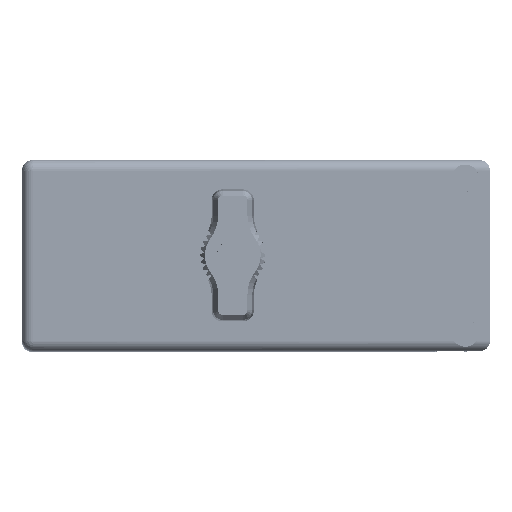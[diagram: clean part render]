
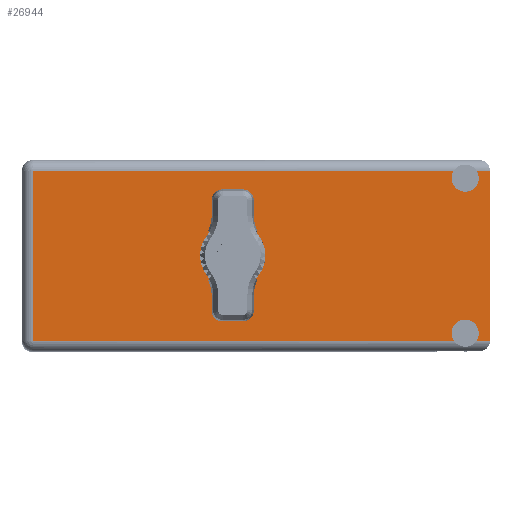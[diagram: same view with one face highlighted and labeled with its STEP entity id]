
A CAD part, top view. The second image highlights one B-rep face of the part: STEP entity #26944.
In plain terms, the highlighted face is planar.
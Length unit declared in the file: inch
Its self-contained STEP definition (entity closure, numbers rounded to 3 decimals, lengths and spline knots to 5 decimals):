
#240 = ORIENTED_EDGE ( 'NONE', *, *, #15233, .F. ) ;
#1198 = CARTESIAN_POINT ( 'NONE',  ( 1.42519, 1.675, -0.547 ) ) ;
#1617 = CARTESIAN_POINT ( 'NONE',  ( 1.499, 1.675, 0.5 ) ) ;
#3322 = CARTESIAN_POINT ( 'NONE',  ( 1.499, 1.675, -0.5 ) ) ;
#3439 = ORIENTED_EDGE ( 'NONE', *, *, #83139, .F. ) ;
#4769 = CARTESIAN_POINT ( 'NONE',  ( 1.659, 1.675, 0.617 ) ) ;
#5890 = LINE ( 'NONE', #4769, #50999 ) ;
#5901 = CARTESIAN_POINT ( 'NONE',  ( 1.42519, 1.675, 0.547 ) ) ;
#5935 = EDGE_CURVE ( 'NONE', #7246, #65026, #33820, .T. ) ;
#6050 = CARTESIAN_POINT ( 'NONE',  ( 0., 1.675, 0.125 ) ) ;
#7246 = VERTEX_POINT ( 'NONE', #82256 ) ;
#9807 = CARTESIAN_POINT ( 'NONE',  ( 1.499, 1.675, -0.4125 ) ) ;
#10256 = PLANE ( 'NONE',  #47088 ) ;
#10401 = DIRECTION ( 'NONE',  ( 0., 1., 0. ) ) ;
#10644 = VECTOR ( 'NONE', #65956, 39.37008 ) ;
#11143 = CARTESIAN_POINT ( 'NONE',  ( 1.659, 1.675, 0.547 ) ) ;
#11753 = DIRECTION ( 'NONE',  ( 0., 1., 0. ) ) ;
#13072 = CIRCLE ( 'NONE', #24403, 0.0875 ) ;
#14106 = DIRECTION ( 'NONE',  ( 0., 0., 1. ) ) ;
#14936 = CARTESIAN_POINT ( 'NONE',  ( -1.289, 1.675, -0.617 ) ) ;
#15233 = EDGE_CURVE ( 'NONE', #57375, #23642, #34557, .T. ) ;
#15489 = CARTESIAN_POINT ( 'NONE',  ( 1.659, 1.675, -0.547 ) ) ;
#16660 = DIRECTION ( 'NONE',  ( 1., 0., 0. ) ) ;
#16990 = CARTESIAN_POINT ( 'NONE',  ( -1.359, 1.675, -0.617 ) ) ;
#17126 = EDGE_CURVE ( 'NONE', #56191, #57375, #13072, .T. ) ;
#18173 = VERTEX_POINT ( 'NONE', #37630 ) ;
#18521 = EDGE_CURVE ( 'NONE', #23300, #18173, #86095, .T. ) ;
#19029 = CARTESIAN_POINT ( 'NONE',  ( 1.499, 1.675, -0.5 ) ) ;
#19061 = CARTESIAN_POINT ( 'NONE',  ( 0., 1.675, 0. ) ) ;
#22151 = CARTESIAN_POINT ( 'NONE',  ( 1.659, 1.675, 0.547 ) ) ;
#22225 = ORIENTED_EDGE ( 'NONE', *, *, #76619, .T. ) ;
#22551 = CARTESIAN_POINT ( 'NONE',  ( 1.659, 1.675, 0.547 ) ) ;
#23282 = EDGE_CURVE ( 'NONE', #18173, #34765, #85781, .T. ) ;
#23300 = VERTEX_POINT ( 'NONE', #86398 ) ;
#23642 = VERTEX_POINT ( 'NONE', #68958 ) ;
#24315 = DIRECTION ( 'NONE',  ( 1., 0., 0. ) ) ;
#24345 = CARTESIAN_POINT ( 'NONE',  ( -1.359, 1.675, -0.547 ) ) ;
#24403 = AXIS2_PLACEMENT_3D ( 'NONE', #3322, #50161, #77026 ) ;
#26257 = ORIENTED_EDGE ( 'NONE', *, *, #17126, .F. ) ;
#26944 = ADVANCED_FACE ( 'NONE', ( #64418, #38084 ), #10256, .T. ) ;
#27658 = CIRCLE ( 'NONE', #44331, 0.125 ) ;
#27825 = DIRECTION ( 'NONE',  ( 0., 0., 1. ) ) ;
#29910 = AXIS2_PLACEMENT_3D ( 'NONE', #19029, #11753, #51320 ) ;
#30744 = ORIENTED_EDGE ( 'NONE', *, *, #5935, .T. ) ;
#31118 = VECTOR ( 'NONE', #16660, 39.37008 ) ;
#31704 = EDGE_CURVE ( 'NONE', #23300, #59989, #43831, .T. ) ;
#31727 = CARTESIAN_POINT ( 'NONE',  ( 1.499, 1.675, 0.5 ) ) ;
#31732 = VERTEX_POINT ( 'NONE', #15489 ) ;
#31738 = VECTOR ( 'NONE', #27825, 39.37008 ) ;
#33820 = LINE ( 'NONE', #14936, #31738 ) ;
#34463 = AXIS2_PLACEMENT_3D ( 'NONE', #1617, #41115, #14106 ) ;
#34557 = CIRCLE ( 'NONE', #29910, 0.0875 ) ;
#34765 = VERTEX_POINT ( 'NONE', #5901 ) ;
#35515 = CIRCLE ( 'NONE', #42344, 0.125 ) ;
#35766 = CARTESIAN_POINT ( 'NONE',  ( 0., 1.675, -0.125 ) ) ;
#37348 = CARTESIAN_POINT ( 'NONE',  ( 0., 1.675, 0. ) ) ;
#37630 = CARTESIAN_POINT ( 'NONE',  ( 1.499, 1.675, 0.4125 ) ) ;
#38084 = FACE_OUTER_BOUND ( 'NONE', #60533, .T. ) ;
#38307 = ORIENTED_EDGE ( 'NONE', *, *, #18521, .F. ) ;
#38422 = DIRECTION ( 'NONE',  ( 0., 1., 0. ) ) ;
#38501 = DIRECTION ( 'NONE',  ( 0., 1., 0. ) ) ;
#38522 = CARTESIAN_POINT ( 'NONE',  ( -1.289, 1.675, 0.547 ) ) ;
#41113 = ORIENTED_EDGE ( 'NONE', *, *, #31704, .T. ) ;
#41115 = DIRECTION ( 'NONE',  ( 0., 1., 0. ) ) ;
#41990 = ORIENTED_EDGE ( 'NONE', *, *, #61314, .T. ) ;
#42344 = AXIS2_PLACEMENT_3D ( 'NONE', #19061, #38422, #79071 ) ;
#42806 = VECTOR ( 'NONE', #24315, 39.37008 ) ;
#43491 = VERTEX_POINT ( 'NONE', #35766 ) ;
#43831 = LINE ( 'NONE', #22551, #31118 ) ;
#44331 = AXIS2_PLACEMENT_3D ( 'NONE', #37348, #10401, #57354 ) ;
#45586 = DIRECTION ( 'NONE',  ( 0., 0., 1. ) ) ;
#46006 = CARTESIAN_POINT ( 'NONE',  ( -1.359, 1.675, -0.547 ) ) ;
#46294 = LINE ( 'NONE', #46006, #10644 ) ;
#46613 = EDGE_CURVE ( 'NONE', #43491, #70451, #27658, .T. ) ;
#46940 = LINE ( 'NONE', #11143, #42806 ) ;
#47088 = AXIS2_PLACEMENT_3D ( 'NONE', #16990, #83171, #76158 ) ;
#48798 = EDGE_LOOP ( 'NONE', ( #3439, #77799 ) ) ;
#50161 = DIRECTION ( 'NONE',  ( 0., 1., 0. ) ) ;
#50999 = VECTOR ( 'NONE', #51064, 39.37008 ) ;
#51064 = DIRECTION ( 'NONE',  ( 0., 0., 1. ) ) ;
#51320 = DIRECTION ( 'NONE',  ( 0., 0., 1. ) ) ;
#53474 = ORIENTED_EDGE ( 'NONE', *, *, #66045, .F. ) ;
#56191 = VERTEX_POINT ( 'NONE', #1198 ) ;
#56848 = VECTOR ( 'NONE', #77896, 39.37008 ) ;
#57354 = DIRECTION ( 'NONE',  ( 0., 0., 1. ) ) ;
#57375 = VERTEX_POINT ( 'NONE', #9807 ) ;
#59989 = VERTEX_POINT ( 'NONE', #22151 ) ;
#60533 = EDGE_LOOP ( 'NONE', ( #41990, #79885, #38307, #41113, #53474, #22225, #240, #26257, #77978, #30744 ) ) ;
#61314 = EDGE_CURVE ( 'NONE', #65026, #34765, #46940, .T. ) ;
#63871 = AXIS2_PLACEMENT_3D ( 'NONE', #31727, #38501, #45586 ) ;
#64418 = FACE_BOUND ( 'NONE', #48798, .T. ) ;
#65026 = VERTEX_POINT ( 'NONE', #38522 ) ;
#65956 = DIRECTION ( 'NONE',  ( -1., 0., 0. ) ) ;
#66045 = EDGE_CURVE ( 'NONE', #31732, #59989, #5890, .T. ) ;
#68958 = CARTESIAN_POINT ( 'NONE',  ( 1.57281, 1.675, -0.547 ) ) ;
#70451 = VERTEX_POINT ( 'NONE', #6050 ) ;
#74549 = LINE ( 'NONE', #24345, #56848 ) ;
#76158 = DIRECTION ( 'NONE',  ( -1., 0., 0. ) ) ;
#76610 = EDGE_CURVE ( 'NONE', #56191, #7246, #74549, .T. ) ;
#76619 = EDGE_CURVE ( 'NONE', #31732, #23642, #46294, .T. ) ;
#77026 = DIRECTION ( 'NONE',  ( 0., 0., 1. ) ) ;
#77799 = ORIENTED_EDGE ( 'NONE', *, *, #46613, .F. ) ;
#77896 = DIRECTION ( 'NONE',  ( -1., 0., 0. ) ) ;
#77978 = ORIENTED_EDGE ( 'NONE', *, *, #76610, .T. ) ;
#79071 = DIRECTION ( 'NONE',  ( 0., 0., 1. ) ) ;
#79885 = ORIENTED_EDGE ( 'NONE', *, *, #23282, .F. ) ;
#82256 = CARTESIAN_POINT ( 'NONE',  ( -1.289, 1.675, -0.547 ) ) ;
#83139 = EDGE_CURVE ( 'NONE', #70451, #43491, #35515, .T. ) ;
#83171 = DIRECTION ( 'NONE',  ( 0., 1., 0. ) ) ;
#85781 = CIRCLE ( 'NONE', #63871, 0.0875 ) ;
#86095 = CIRCLE ( 'NONE', #34463, 0.0875 ) ;
#86398 = CARTESIAN_POINT ( 'NONE',  ( 1.57281, 1.675, 0.547 ) ) ;
